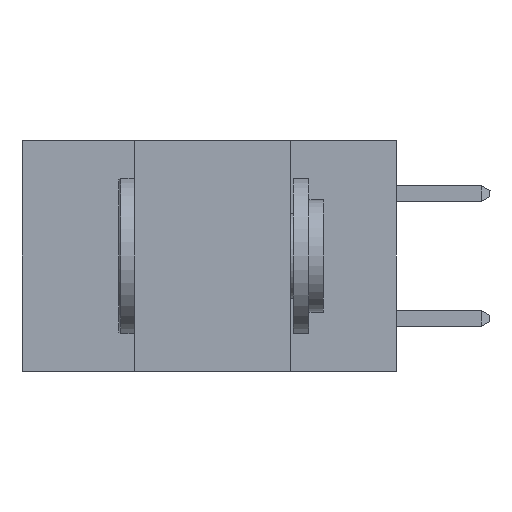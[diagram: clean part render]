
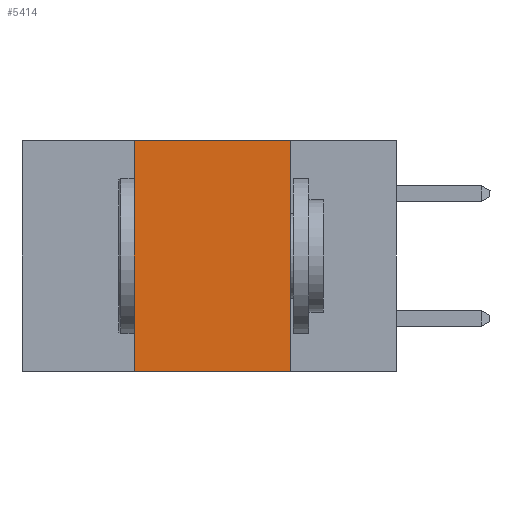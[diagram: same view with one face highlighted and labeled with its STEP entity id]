
A CAD part, left-side view. The second image highlights one B-rep face of the part: STEP entity #5414.
In plain terms, the highlighted planar face has unit normal (-1, 0, 0).
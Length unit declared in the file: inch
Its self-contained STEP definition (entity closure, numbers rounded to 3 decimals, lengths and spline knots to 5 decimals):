
#446 = ORIENTED_EDGE ( 'NONE', *, *, #17566, .T. ) ;
#944 = VECTOR ( 'NONE', #13379, 39.37008 ) ;
#1179 = EDGE_LOOP ( 'NONE', ( #10978, #13768, #19678, #446 ) ) ;
#1399 = LINE ( 'NONE', #9521, #20334 ) ;
#1401 = VERTEX_POINT ( 'NONE', #16306 ) ;
#5414 = ADVANCED_FACE ( 'NONE', ( #14785 ), #14970, .F. ) ;
#6409 = VECTOR ( 'NONE', #10081, 39.37008 ) ;
#7806 = CARTESIAN_POINT ( 'NONE',  ( 0., 0.42, 0. ) ) ;
#8402 = CARTESIAN_POINT ( 'NONE',  ( 0., 0.17, 0. ) ) ;
#8726 = VERTEX_POINT ( 'NONE', #21347 ) ;
#9521 = CARTESIAN_POINT ( 'NONE',  ( 0., 0.6, -0.37 ) ) ;
#10081 = DIRECTION ( 'NONE',  ( 0., -1., 0. ) ) ;
#10380 = EDGE_CURVE ( 'NONE', #20279, #8726, #10454, .T. ) ;
#10454 = LINE ( 'NONE', #20489, #14647 ) ;
#10978 = ORIENTED_EDGE ( 'NONE', *, *, #10380, .F. ) ;
#11233 = LINE ( 'NONE', #18911, #6409 ) ;
#11671 = CARTESIAN_POINT ( 'NONE',  ( 0., 0.42, -0.37 ) ) ;
#13379 = DIRECTION ( 'NONE',  ( 0., 0., 1. ) ) ;
#13768 = ORIENTED_EDGE ( 'NONE', *, *, #13978, .F. ) ;
#13978 = EDGE_CURVE ( 'NONE', #16368, #20279, #11233, .T. ) ;
#14647 = VECTOR ( 'NONE', #22274, 39.37008 ) ;
#14763 = DIRECTION ( 'NONE',  ( 0., 0., -1. ) ) ;
#14785 = FACE_OUTER_BOUND ( 'NONE', #1179, .T. ) ;
#14786 = DIRECTION ( 'NONE',  ( 1., 0., 0. ) ) ;
#14970 = PLANE ( 'NONE',  #15134 ) ;
#14976 = CARTESIAN_POINT ( 'NONE',  ( 0., 0.6, 0. ) ) ;
#15134 = AXIS2_PLACEMENT_3D ( 'NONE', #14976, #14786, #14763 ) ;
#15173 = EDGE_CURVE ( 'NONE', #1401, #16368, #23551, .T. ) ;
#16306 = CARTESIAN_POINT ( 'NONE',  ( 0., 0.42, -0.37 ) ) ;
#16368 = VERTEX_POINT ( 'NONE', #7806 ) ;
#17566 = EDGE_CURVE ( 'NONE', #1401, #8726, #1399, .T. ) ;
#18911 = CARTESIAN_POINT ( 'NONE',  ( 0., 0.6, 0. ) ) ;
#19678 = ORIENTED_EDGE ( 'NONE', *, *, #15173, .F. ) ;
#20161 = DIRECTION ( 'NONE',  ( 0., -1., 0. ) ) ;
#20279 = VERTEX_POINT ( 'NONE', #8402 ) ;
#20334 = VECTOR ( 'NONE', #20161, 39.37008 ) ;
#20489 = CARTESIAN_POINT ( 'NONE',  ( 0., 0.17, -0.37 ) ) ;
#21347 = CARTESIAN_POINT ( 'NONE',  ( 0., 0.17, -0.37 ) ) ;
#22274 = DIRECTION ( 'NONE',  ( 0., 0., -1. ) ) ;
#23551 = LINE ( 'NONE', #11671, #944 ) ;
